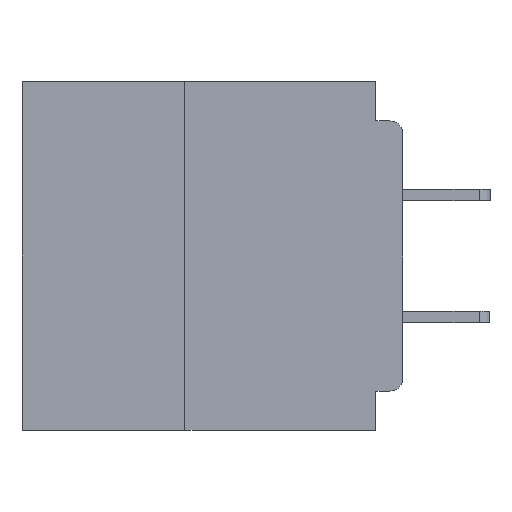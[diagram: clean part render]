
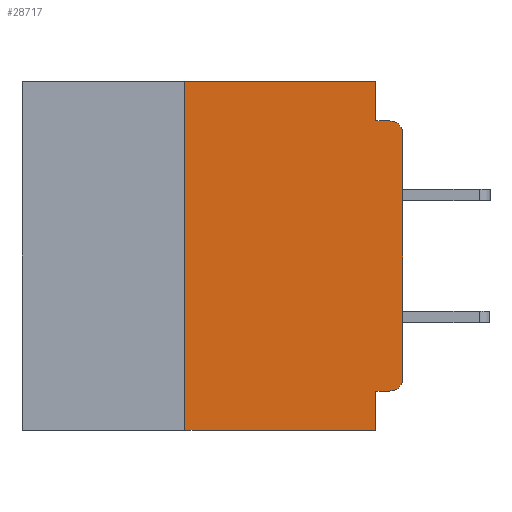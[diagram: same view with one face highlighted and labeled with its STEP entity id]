
A CAD part, left-side view. The second image highlights one B-rep face of the part: STEP entity #28717.
In plain terms, the highlighted planar face has unit normal (-1, 0, 0).
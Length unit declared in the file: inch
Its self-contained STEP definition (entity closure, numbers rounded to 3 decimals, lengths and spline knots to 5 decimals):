
#626 = DIRECTION ( 'NONE',  ( 0., 0., -1. ) ) ;
#727 = ORIENTED_EDGE ( 'NONE', *, *, #20773, .F. ) ;
#752 = DIRECTION ( 'NONE',  ( 0., 0., -1. ) ) ;
#1308 = LINE ( 'NONE', #43929, #22449 ) ;
#1855 = LINE ( 'NONE', #29736, #40139 ) ;
#2062 = CARTESIAN_POINT ( 'NONE',  ( 0., 0.031, -0.4 ) ) ;
#4158 = ORIENTED_EDGE ( 'NONE', *, *, #26247, .F. ) ;
#5446 = ORIENTED_EDGE ( 'NONE', *, *, #21580, .F. ) ;
#5734 = CARTESIAN_POINT ( 'NONE',  ( 0., 0., 0. ) ) ;
#6003 = VERTEX_POINT ( 'NONE', #24890 ) ;
#6063 = ORIENTED_EDGE ( 'NONE', *, *, #40155, .F. ) ;
#6207 = VECTOR ( 'NONE', #9516, 39.37008 ) ;
#6878 = VERTEX_POINT ( 'NONE', #44488 ) ;
#7147 = CARTESIAN_POINT ( 'NONE',  ( 0., 0.031, 0. ) ) ;
#7453 = DIRECTION ( 'NONE',  ( 0., 1., 0. ) ) ;
#8425 = CARTESIAN_POINT ( 'NONE',  ( 0., 0.437, 0. ) ) ;
#9322 = CARTESIAN_POINT ( 'NONE',  ( 0., 0., -0.34 ) ) ;
#9516 = DIRECTION ( 'NONE',  ( 0., 0., 1. ) ) ;
#9676 = VERTEX_POINT ( 'NONE', #9322 ) ;
#10666 = VECTOR ( 'NONE', #23569, 39.37008 ) ;
#10981 = FACE_OUTER_BOUND ( 'NONE', #37795, .T. ) ;
#12151 = DIRECTION ( 'NONE',  ( 0., -1., 0. ) ) ;
#14754 = LINE ( 'NONE', #8425, #33289 ) ;
#15022 = EDGE_CURVE ( 'NONE', #6003, #46998, #1308, .T. ) ;
#15175 = DIRECTION ( 'NONE',  ( 0., 0., -1. ) ) ;
#15301 = CARTESIAN_POINT ( 'NONE',  ( 0., 0.031, -0.045 ) ) ;
#17174 = CARTESIAN_POINT ( 'NONE',  ( 0., 0.015, -0.34 ) ) ;
#17589 = CARTESIAN_POINT ( 'NONE',  ( 0., 0.25, -0.4 ) ) ;
#18930 = CARTESIAN_POINT ( 'NONE',  ( 0., 0.25, 0. ) ) ;
#18955 = ORIENTED_EDGE ( 'NONE', *, *, #25254, .F. ) ;
#19827 = CARTESIAN_POINT ( 'NONE',  ( 0., 0., -0.045 ) ) ;
#19996 = ORIENTED_EDGE ( 'NONE', *, *, #15022, .T. ) ;
#20042 = CARTESIAN_POINT ( 'NONE',  ( 0., 0.031, -0.355 ) ) ;
#20773 = EDGE_CURVE ( 'NONE', #35980, #46998, #40790, .T. ) ;
#20880 = VERTEX_POINT ( 'NONE', #25138 ) ;
#20979 = DIRECTION ( 'NONE',  ( 0., 0., -1. ) ) ;
#21359 = LINE ( 'NONE', #17589, #40825 ) ;
#21426 = EDGE_CURVE ( 'NONE', #20880, #35980, #1855, .T. ) ;
#21580 = EDGE_CURVE ( 'NONE', #31961, #40074, #14754, .T. ) ;
#22009 = DIRECTION ( 'NONE',  ( 0., -1., 0. ) ) ;
#22408 = ORIENTED_EDGE ( 'NONE', *, *, #41133, .T. ) ;
#22449 = VECTOR ( 'NONE', #22009, 39.37008 ) ;
#22668 = AXIS2_PLACEMENT_3D ( 'NONE', #17174, #42933, #20979 ) ;
#22972 = VERTEX_POINT ( 'NONE', #43008 ) ;
#23126 = DIRECTION ( 'NONE',  ( 1., 0., 0. ) ) ;
#23252 = DIRECTION ( 'NONE',  ( -1., 0., 0. ) ) ;
#23569 = DIRECTION ( 'NONE',  ( 0., -1., 0. ) ) ;
#24382 = CARTESIAN_POINT ( 'NONE',  ( 0., 0.031, -0.4 ) ) ;
#24407 = EDGE_CURVE ( 'NONE', #6878, #22972, #46571, .T. ) ;
#24890 = CARTESIAN_POINT ( 'NONE',  ( 0., 0.25, -0.4 ) ) ;
#25138 = CARTESIAN_POINT ( 'NONE',  ( 0., 0.015, -0.355 ) ) ;
#25254 = EDGE_CURVE ( 'NONE', #6003, #31961, #21359, .T. ) ;
#26247 = EDGE_CURVE ( 'NONE', #41811, #22972, #31639, .T. ) ;
#26678 = CARTESIAN_POINT ( 'NONE',  ( 0., 0.437, 0. ) ) ;
#28225 = DIRECTION ( 'NONE',  ( 0., 0., -1. ) ) ;
#28717 = ADVANCED_FACE ( 'NONE', ( #10981 ), #37656, .F. ) ;
#28810 = DIRECTION ( 'NONE',  ( 0., 0., 1. ) ) ;
#29005 = AXIS2_PLACEMENT_3D ( 'NONE', #26678, #23126, #626 ) ;
#29692 = ORIENTED_EDGE ( 'NONE', *, *, #24407, .T. ) ;
#29736 = CARTESIAN_POINT ( 'NONE',  ( 0., 0., -0.355 ) ) ;
#29761 = AXIS2_PLACEMENT_3D ( 'NONE', #45159, #23252, #752 ) ;
#31265 = VECTOR ( 'NONE', #15175, 39.37008 ) ;
#31639 = LINE ( 'NONE', #19827, #10666 ) ;
#31961 = VERTEX_POINT ( 'NONE', #18930 ) ;
#32251 = VECTOR ( 'NONE', #28225, 39.37008 ) ;
#33289 = VECTOR ( 'NONE', #12151, 39.37008 ) ;
#34650 = ORIENTED_EDGE ( 'NONE', *, *, #42705, .T. ) ;
#35734 = LINE ( 'NONE', #5734, #6207 ) ;
#35980 = VERTEX_POINT ( 'NONE', #20042 ) ;
#37656 = PLANE ( 'NONE',  #29005 ) ;
#37795 = EDGE_LOOP ( 'NONE', ( #22408, #29692, #4158, #6063, #5446, #18955, #19996, #727, #47248, #34650 ) ) ;
#40074 = VERTEX_POINT ( 'NONE', #7147 ) ;
#40139 = VECTOR ( 'NONE', #7453, 39.37008 ) ;
#40155 = EDGE_CURVE ( 'NONE', #40074, #41811, #40919, .T. ) ;
#40790 = LINE ( 'NONE', #2062, #32251 ) ;
#40825 = VECTOR ( 'NONE', #28810, 39.37008 ) ;
#40919 = LINE ( 'NONE', #44404, #31265 ) ;
#41133 = EDGE_CURVE ( 'NONE', #9676, #6878, #35734, .T. ) ;
#41811 = VERTEX_POINT ( 'NONE', #15301 ) ;
#42705 = EDGE_CURVE ( 'NONE', #20880, #9676, #45269, .T. ) ;
#42933 = DIRECTION ( 'NONE',  ( -1., 0., 0. ) ) ;
#43008 = CARTESIAN_POINT ( 'NONE',  ( 0., 0.015, -0.045 ) ) ;
#43929 = CARTESIAN_POINT ( 'NONE',  ( 0., 0.437, -0.4 ) ) ;
#44404 = CARTESIAN_POINT ( 'NONE',  ( 0., 0.031, 0. ) ) ;
#44488 = CARTESIAN_POINT ( 'NONE',  ( 0., 0., -0.06 ) ) ;
#45159 = CARTESIAN_POINT ( 'NONE',  ( 0., 0.015, -0.06 ) ) ;
#45269 = CIRCLE ( 'NONE', #22668, 0.015 ) ;
#46571 = CIRCLE ( 'NONE', #29761, 0.015 ) ;
#46998 = VERTEX_POINT ( 'NONE', #24382 ) ;
#47248 = ORIENTED_EDGE ( 'NONE', *, *, #21426, .F. ) ;
